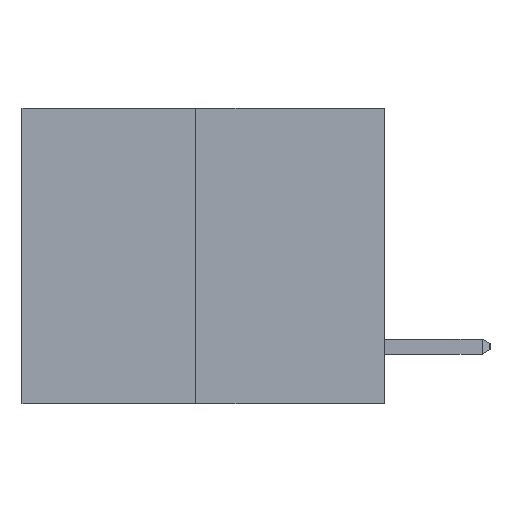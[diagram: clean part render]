
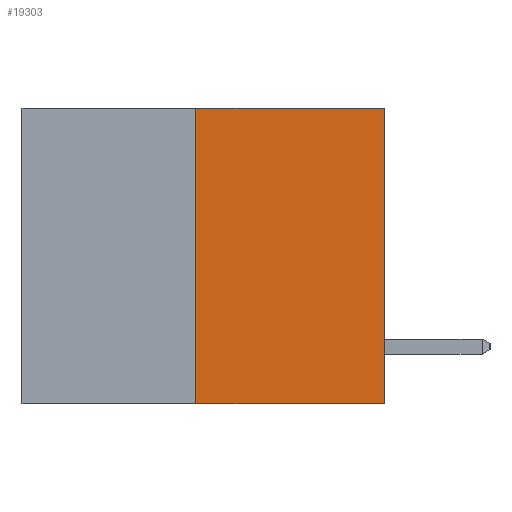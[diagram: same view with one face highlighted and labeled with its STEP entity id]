
A CAD part, left-side view. The second image highlights one B-rep face of the part: STEP entity #19303.
In plain terms, the highlighted planar face has unit normal (-1, 0, 0).
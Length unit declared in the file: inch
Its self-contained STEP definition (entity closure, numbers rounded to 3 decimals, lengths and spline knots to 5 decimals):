
#1620 = ORIENTED_EDGE ( 'NONE', *, *, #16949, .T. ) ;
#2104 = EDGE_CURVE ( 'NONE', #7608, #18563, #13203, .T. ) ;
#2480 = EDGE_LOOP ( 'NONE', ( #6864, #1620, #20915, #4636 ) ) ;
#4193 = CARTESIAN_POINT ( 'NONE',  ( 0., 0.6, 0. ) ) ;
#4341 = VERTEX_POINT ( 'NONE', #16235 ) ;
#4636 = ORIENTED_EDGE ( 'NONE', *, *, #2104, .F. ) ;
#6189 = FACE_OUTER_BOUND ( 'NONE', #2480, .T. ) ;
#6864 = ORIENTED_EDGE ( 'NONE', *, *, #13845, .F. ) ;
#7284 = DIRECTION ( 'NONE',  ( 0., -1., 0. ) ) ;
#7608 = VERTEX_POINT ( 'NONE', #21995 ) ;
#7764 = DIRECTION ( 'NONE',  ( 0., -1., 0. ) ) ;
#7919 = DIRECTION ( 'NONE',  ( 0., 0., -1. ) ) ;
#8055 = VECTOR ( 'NONE', #12386, 39.37008 ) ;
#8157 = DIRECTION ( 'NONE',  ( 1., 0., 0. ) ) ;
#9742 = CARTESIAN_POINT ( 'NONE',  ( 0., 0.6, 0. ) ) ;
#10235 = CARTESIAN_POINT ( 'NONE',  ( 0., 0.312, -0.49 ) ) ;
#12386 = DIRECTION ( 'NONE',  ( 0., 0., 1. ) ) ;
#12529 = VECTOR ( 'NONE', #7284, 39.37008 ) ;
#13203 = LINE ( 'NONE', #9742, #18382 ) ;
#13394 = CARTESIAN_POINT ( 'NONE',  ( 0., 0., 0. ) ) ;
#13845 = EDGE_CURVE ( 'NONE', #14732, #7608, #14768, .T. ) ;
#14486 = CARTESIAN_POINT ( 'NONE',  ( 0., 0.6, -0.49 ) ) ;
#14732 = VERTEX_POINT ( 'NONE', #10235 ) ;
#14768 = LINE ( 'NONE', #21608, #8055 ) ;
#16235 = CARTESIAN_POINT ( 'NONE',  ( 0., 0., -0.49 ) ) ;
#16450 = CARTESIAN_POINT ( 'NONE',  ( 0., 0., 0. ) ) ;
#16612 = LINE ( 'NONE', #16450, #23508 ) ;
#16949 = EDGE_CURVE ( 'NONE', #14732, #4341, #22377, .T. ) ;
#18382 = VECTOR ( 'NONE', #7764, 39.37008 ) ;
#18471 = DIRECTION ( 'NONE',  ( 0., 0., 1. ) ) ;
#18563 = VERTEX_POINT ( 'NONE', #13394 ) ;
#19303 = ADVANCED_FACE ( 'NONE', ( #6189 ), #19306, .F. ) ;
#19306 = PLANE ( 'NONE',  #21591 ) ;
#20915 = ORIENTED_EDGE ( 'NONE', *, *, #23133, .T. ) ;
#21591 = AXIS2_PLACEMENT_3D ( 'NONE', #4193, #8157, #7919 ) ;
#21608 = CARTESIAN_POINT ( 'NONE',  ( 0., 0.312, -0.49 ) ) ;
#21995 = CARTESIAN_POINT ( 'NONE',  ( 0., 0.312, 0. ) ) ;
#22377 = LINE ( 'NONE', #14486, #12529 ) ;
#23133 = EDGE_CURVE ( 'NONE', #4341, #18563, #16612, .T. ) ;
#23508 = VECTOR ( 'NONE', #18471, 39.37008 ) ;
